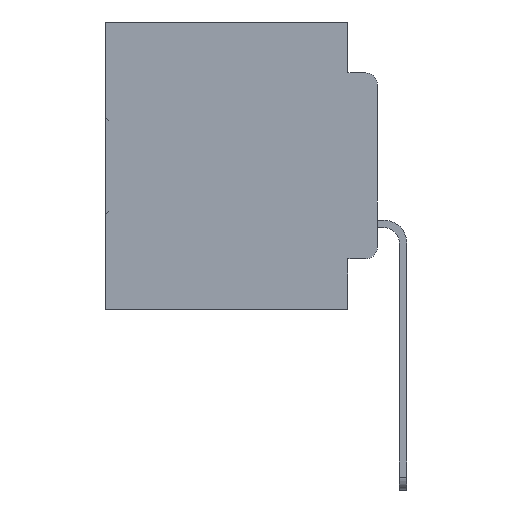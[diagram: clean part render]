
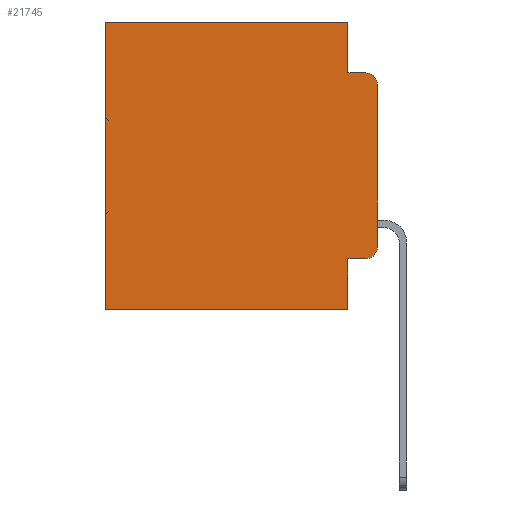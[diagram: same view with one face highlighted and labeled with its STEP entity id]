
A CAD part, left-side view. The second image highlights one B-rep face of the part: STEP entity #21745.
In plain terms, the highlighted planar face has unit normal (-1, 0, 0).
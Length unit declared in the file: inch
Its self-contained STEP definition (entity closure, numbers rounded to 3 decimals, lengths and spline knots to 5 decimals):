
#147 = DIRECTION ( 'NONE',  ( 0., 0., -1. ) ) ;
#936 = EDGE_CURVE ( 'NONE', #33105, #30667, #33100, .T. ) ;
#1039 = CARTESIAN_POINT ( 'NONE',  ( 0.298, 0., -0.1085 ) ) ;
#1290 = CARTESIAN_POINT ( 'NONE',  ( 0.298, 0.473, -0.5 ) ) ;
#1409 = CARTESIAN_POINT ( 'NONE',  ( 0.298, 0.051, -0.5 ) ) ;
#2174 = CARTESIAN_POINT ( 'NONE',  ( 0.298, 0.473, 0. ) ) ;
#2529 = VECTOR ( 'NONE', #10398, 39.37008 ) ;
#2718 = LINE ( 'NONE', #3314, #30086 ) ;
#2752 = EDGE_CURVE ( 'NONE', #12892, #29188, #4165, .T. ) ;
#3314 = CARTESIAN_POINT ( 'NONE',  ( 0.298, 0.051, -0.4115 ) ) ;
#3511 = DIRECTION ( 'NONE',  ( 0., 1., 0. ) ) ;
#3695 = VERTEX_POINT ( 'NONE', #1290 ) ;
#3770 = VECTOR ( 'NONE', #9521, 39.37008 ) ;
#4165 = CIRCLE ( 'NONE', #23287, 0.02 ) ;
#4167 = AXIS2_PLACEMENT_3D ( 'NONE', #23140, #7218, #25737 ) ;
#4670 = CARTESIAN_POINT ( 'NONE',  ( 0.298, 0.051, -0.4115 ) ) ;
#5675 = LINE ( 'NONE', #13776, #19900 ) ;
#5722 = VERTEX_POINT ( 'NONE', #4670 ) ;
#5796 = CARTESIAN_POINT ( 'NONE',  ( 0.298, 0.02, -0.4115 ) ) ;
#6168 = DIRECTION ( 'NONE',  ( 0., 0., -1. ) ) ;
#6709 = CARTESIAN_POINT ( 'NONE',  ( 0.298, 0., -0.5 ) ) ;
#6805 = CARTESIAN_POINT ( 'NONE',  ( 0.298, 0.051, -0.0885 ) ) ;
#6818 = DIRECTION ( 'NONE',  ( 0., 1., 0. ) ) ;
#7218 = DIRECTION ( 'NONE',  ( -1., 0., 0. ) ) ;
#7672 = CARTESIAN_POINT ( 'NONE',  ( 0.298, 0.051, 0. ) ) ;
#7856 = DIRECTION ( 'NONE',  ( 0., 0., -1. ) ) ;
#8707 = VERTEX_POINT ( 'NONE', #1409 ) ;
#9143 = CARTESIAN_POINT ( 'NONE',  ( 0.298, 0.051, 0. ) ) ;
#9521 = DIRECTION ( 'NONE',  ( 0., -1., 0. ) ) ;
#10398 = DIRECTION ( 'NONE',  ( 0., 0., -1. ) ) ;
#10576 = VERTEX_POINT ( 'NONE', #1039 ) ;
#11088 = VECTOR ( 'NONE', #6818, 39.37008 ) ;
#11239 = DIRECTION ( 'NONE',  ( -1., 0., 0. ) ) ;
#11282 = CARTESIAN_POINT ( 'NONE',  ( 0.298, 0.02, -0.3915 ) ) ;
#11897 = ORIENTED_EDGE ( 'NONE', *, *, #2752, .T. ) ;
#12892 = VERTEX_POINT ( 'NONE', #5796 ) ;
#13524 = EDGE_CURVE ( 'NONE', #10576, #29188, #5675, .T. ) ;
#13776 = CARTESIAN_POINT ( 'NONE',  ( 0.298, 0., 0. ) ) ;
#15142 = EDGE_CURVE ( 'NONE', #8707, #3695, #25125, .T. ) ;
#15763 = VECTOR ( 'NONE', #3511, 39.37008 ) ;
#16841 = CARTESIAN_POINT ( 'NONE',  ( 0.298, 0.051, -0.0885 ) ) ;
#16948 = LINE ( 'NONE', #7672, #2529 ) ;
#17848 = ORIENTED_EDGE ( 'NONE', *, *, #25801, .T. ) ;
#18233 = DIRECTION ( 'NONE',  ( 0., 0., -1. ) ) ;
#18335 = EDGE_CURVE ( 'NONE', #5722, #12892, #2718, .T. ) ;
#18870 = AXIS2_PLACEMENT_3D ( 'NONE', #33925, #23777, #7856 ) ;
#19210 = CARTESIAN_POINT ( 'NONE',  ( 0.298, 0.051, 0. ) ) ;
#19461 = VECTOR ( 'NONE', #147, 39.37008 ) ;
#19639 = CARTESIAN_POINT ( 'NONE',  ( 0.298, 0., 0. ) ) ;
#19778 = EDGE_CURVE ( 'NONE', #10576, #26756, #25166, .T. ) ;
#19900 = VECTOR ( 'NONE', #29386, 39.37008 ) ;
#21141 = PLANE ( 'NONE',  #18870 ) ;
#21528 = EDGE_CURVE ( 'NONE', #30667, #26756, #25041, .T. ) ;
#21715 = VERTEX_POINT ( 'NONE', #2174 ) ;
#21745 = ADVANCED_FACE ( 'NONE', ( #23829 ), #21141, .F. ) ;
#23122 = ORIENTED_EDGE ( 'NONE', *, *, #19778, .T. ) ;
#23140 = CARTESIAN_POINT ( 'NONE',  ( 0.298, 0.02, -0.1085 ) ) ;
#23287 = AXIS2_PLACEMENT_3D ( 'NONE', #11282, #11239, #6168 ) ;
#23777 = DIRECTION ( 'NONE',  ( 1., 0., 0. ) ) ;
#23829 = FACE_OUTER_BOUND ( 'NONE', #23970, .T. ) ;
#23970 = EDGE_LOOP ( 'NONE', ( #31522, #23122, #27709, #33941, #17848, #24914, #32415, #32339, #33965, #11897 ) ) ;
#24914 = ORIENTED_EDGE ( 'NONE', *, *, #26151, .T. ) ;
#25041 = LINE ( 'NONE', #6805, #3770 ) ;
#25125 = LINE ( 'NONE', #6709, #11088 ) ;
#25166 = CIRCLE ( 'NONE', #4167, 0.02 ) ;
#25737 = DIRECTION ( 'NONE',  ( 0., 0., -1. ) ) ;
#25801 = EDGE_CURVE ( 'NONE', #33105, #21715, #29584, .T. ) ;
#26085 = CARTESIAN_POINT ( 'NONE',  ( 0.298, 0.473, 0. ) ) ;
#26151 = EDGE_CURVE ( 'NONE', #21715, #3695, #26774, .T. ) ;
#26756 = VERTEX_POINT ( 'NONE', #32278 ) ;
#26774 = LINE ( 'NONE', #26085, #33529 ) ;
#27155 = DIRECTION ( 'NONE',  ( 0., -1., 0. ) ) ;
#27404 = CARTESIAN_POINT ( 'NONE',  ( 0.298, 0., -0.3915 ) ) ;
#27709 = ORIENTED_EDGE ( 'NONE', *, *, #21528, .F. ) ;
#29188 = VERTEX_POINT ( 'NONE', #27404 ) ;
#29386 = DIRECTION ( 'NONE',  ( 0., 0., -1. ) ) ;
#29584 = LINE ( 'NONE', #19639, #15763 ) ;
#30086 = VECTOR ( 'NONE', #27155, 39.37008 ) ;
#30442 = EDGE_CURVE ( 'NONE', #5722, #8707, #16948, .T. ) ;
#30667 = VERTEX_POINT ( 'NONE', #16841 ) ;
#31522 = ORIENTED_EDGE ( 'NONE', *, *, #13524, .F. ) ;
#32278 = CARTESIAN_POINT ( 'NONE',  ( 0.298, 0.02, -0.0885 ) ) ;
#32339 = ORIENTED_EDGE ( 'NONE', *, *, #30442, .F. ) ;
#32415 = ORIENTED_EDGE ( 'NONE', *, *, #15142, .F. ) ;
#33100 = LINE ( 'NONE', #19210, #19461 ) ;
#33105 = VERTEX_POINT ( 'NONE', #9143 ) ;
#33529 = VECTOR ( 'NONE', #18233, 39.37008 ) ;
#33925 = CARTESIAN_POINT ( 'NONE',  ( 0.298, 0., 0. ) ) ;
#33941 = ORIENTED_EDGE ( 'NONE', *, *, #936, .F. ) ;
#33965 = ORIENTED_EDGE ( 'NONE', *, *, #18335, .T. ) ;
